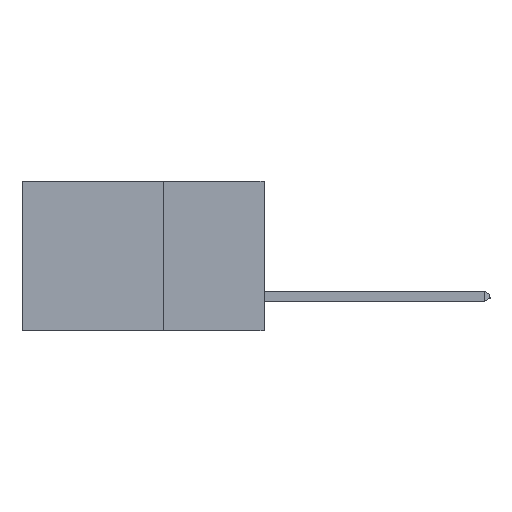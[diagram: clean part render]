
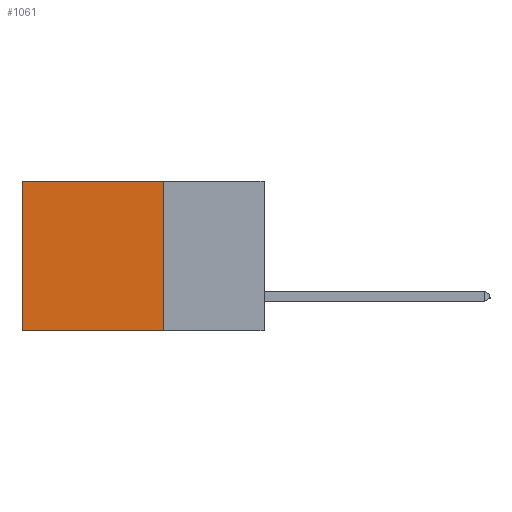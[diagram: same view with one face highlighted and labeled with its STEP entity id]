
A CAD part, left-side view. The second image highlights one B-rep face of the part: STEP entity #1061.
In plain terms, the highlighted planar face has unit normal (-1, 0, 0).
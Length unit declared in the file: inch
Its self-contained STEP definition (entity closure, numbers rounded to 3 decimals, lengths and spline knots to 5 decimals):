
#499 = DIRECTION ( 'NONE',  ( 0., 0., -1. ) ) ;
#904 = LINE ( 'NONE', #3843, #11762 ) ;
#1061 = ADVANCED_FACE ( 'NONE', ( #6782 ), #6231, .F. ) ;
#1536 = DIRECTION ( 'NONE',  ( 0., 0., -1. ) ) ;
#1774 = VECTOR ( 'NONE', #4727, 39.37008 ) ;
#1999 = VERTEX_POINT ( 'NONE', #5064 ) ;
#2388 = EDGE_LOOP ( 'NONE', ( #5705, #5719, #5754, #5766 ) ) ;
#2755 = EDGE_CURVE ( 'NONE', #3985, #1999, #3561, .T. ) ;
#2817 = EDGE_CURVE ( 'NONE', #3985, #8582, #11477, .T. ) ;
#3153 = CARTESIAN_POINT ( 'NONE',  ( 0.298, 0.25, -0.37 ) ) ;
#3561 = LINE ( 'NONE', #8353, #11802 ) ;
#3771 = CARTESIAN_POINT ( 'NONE',  ( 0.298, 0.6, -0.37 ) ) ;
#3843 = CARTESIAN_POINT ( 'NONE',  ( 0.298, 0.6, 0. ) ) ;
#3920 = DIRECTION ( 'NONE',  ( 0., 0., -1. ) ) ;
#3949 = DIRECTION ( 'NONE',  ( 1., 0., 0. ) ) ;
#3985 = VERTEX_POINT ( 'NONE', #6077 ) ;
#4655 = LINE ( 'NONE', #11187, #1774 ) ;
#4727 = DIRECTION ( 'NONE',  ( 0., 1., 0. ) ) ;
#4817 = AXIS2_PLACEMENT_3D ( 'NONE', #7805, #3949, #1536 ) ;
#5064 = CARTESIAN_POINT ( 'NONE',  ( 0.298, 0.6, 0. ) ) ;
#5705 = ORIENTED_EDGE ( 'NONE', *, *, #11324, .T. ) ;
#5719 = ORIENTED_EDGE ( 'NONE', *, *, #7921, .F. ) ;
#5754 = ORIENTED_EDGE ( 'NONE', *, *, #2817, .F. ) ;
#5766 = ORIENTED_EDGE ( 'NONE', *, *, #2755, .T. ) ;
#6077 = CARTESIAN_POINT ( 'NONE',  ( 0.298, 0.25, 0. ) ) ;
#6231 = PLANE ( 'NONE',  #4817 ) ;
#6782 = FACE_OUTER_BOUND ( 'NONE', #2388, .T. ) ;
#7805 = CARTESIAN_POINT ( 'NONE',  ( 0.298, 0.25, 0. ) ) ;
#7921 = EDGE_CURVE ( 'NONE', #8582, #12630, #4655, .T. ) ;
#8353 = CARTESIAN_POINT ( 'NONE',  ( 0.298, 0.25, 0. ) ) ;
#8582 = VERTEX_POINT ( 'NONE', #3153 ) ;
#9613 = CARTESIAN_POINT ( 'NONE',  ( 0.298, 0.25, 0. ) ) ;
#11187 = CARTESIAN_POINT ( 'NONE',  ( 0.298, 0.25, -0.37 ) ) ;
#11299 = DIRECTION ( 'NONE',  ( 0., 1., 0. ) ) ;
#11324 = EDGE_CURVE ( 'NONE', #1999, #12630, #904, .T. ) ;
#11477 = LINE ( 'NONE', #9613, #13939 ) ;
#11762 = VECTOR ( 'NONE', #499, 39.37008 ) ;
#11802 = VECTOR ( 'NONE', #11299, 39.37008 ) ;
#12630 = VERTEX_POINT ( 'NONE', #3771 ) ;
#13939 = VECTOR ( 'NONE', #3920, 39.37008 ) ;
